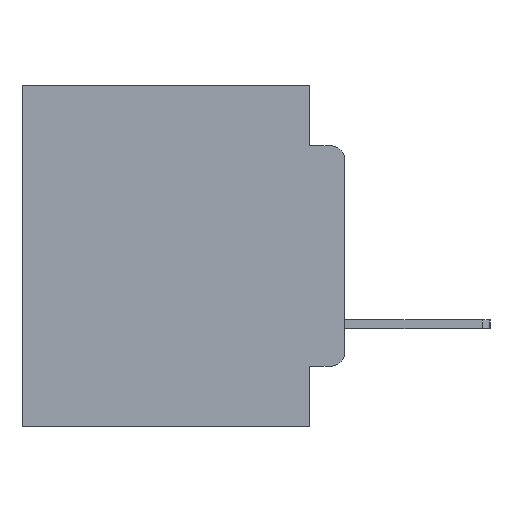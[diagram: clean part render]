
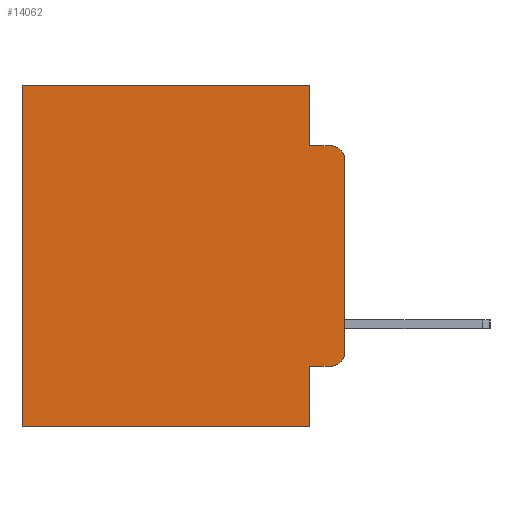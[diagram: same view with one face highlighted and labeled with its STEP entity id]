
A CAD part, left-side view. The second image highlights one B-rep face of the part: STEP entity #14062.
In plain terms, the highlighted planar face has unit normal (-1, 0, 0).
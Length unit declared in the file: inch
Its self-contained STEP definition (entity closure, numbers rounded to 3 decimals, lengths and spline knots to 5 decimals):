
#176 = VERTEX_POINT ( 'NONE', #15971 ) ;
#341 = LINE ( 'NONE', #25611, #21299 ) ;
#705 = EDGE_LOOP ( 'NONE', ( #4758, #1795, #12460, #17952, #14075, #7537, #6541, #7168, #8630, #8923 ) ) ;
#963 = CARTESIAN_POINT ( 'NONE',  ( 0.298, 0.051, -0.0885 ) ) ;
#1400 = EDGE_CURVE ( 'NONE', #21096, #8493, #10377, .T. ) ;
#1471 = CARTESIAN_POINT ( 'NONE',  ( 0.298, 0., -0.3915 ) ) ;
#1538 = DIRECTION ( 'NONE',  ( 0., 0., -1. ) ) ;
#1795 = ORIENTED_EDGE ( 'NONE', *, *, #18095, .T. ) ;
#2127 = DIRECTION ( 'NONE',  ( 0., -1., 0. ) ) ;
#2329 = VECTOR ( 'NONE', #8369, 39.37008 ) ;
#3346 = EDGE_CURVE ( 'NONE', #5875, #17686, #341, .T. ) ;
#3834 = CARTESIAN_POINT ( 'NONE',  ( 0.298, 0.473, 0. ) ) ;
#4711 = VECTOR ( 'NONE', #16511, 39.37008 ) ;
#4758 = ORIENTED_EDGE ( 'NONE', *, *, #12204, .F. ) ;
#5013 = DIRECTION ( 'NONE',  ( -1., 0., 0. ) ) ;
#5567 = LINE ( 'NONE', #6428, #20324 ) ;
#5639 = VECTOR ( 'NONE', #13535, 39.37008 ) ;
#5875 = VERTEX_POINT ( 'NONE', #3834 ) ;
#6010 = PLANE ( 'NONE',  #20145 ) ;
#6085 = CARTESIAN_POINT ( 'NONE',  ( 0.298, 0., 0. ) ) ;
#6158 = CARTESIAN_POINT ( 'NONE',  ( 0.298, 0.473, -0.5 ) ) ;
#6428 = CARTESIAN_POINT ( 'NONE',  ( 0.298, 0., -0.5 ) ) ;
#6541 = ORIENTED_EDGE ( 'NONE', *, *, #20149, .F. ) ;
#7168 = ORIENTED_EDGE ( 'NONE', *, *, #1400, .F. ) ;
#7441 = VECTOR ( 'NONE', #20025, 39.37008 ) ;
#7537 = ORIENTED_EDGE ( 'NONE', *, *, #3346, .T. ) ;
#8031 = CARTESIAN_POINT ( 'NONE',  ( 0.298, 0., -0.1085 ) ) ;
#8080 = LINE ( 'NONE', #6085, #2329 ) ;
#8151 = CARTESIAN_POINT ( 'NONE',  ( 0.298, 0., 0. ) ) ;
#8369 = DIRECTION ( 'NONE',  ( 0., 1., 0. ) ) ;
#8493 = VERTEX_POINT ( 'NONE', #16920 ) ;
#8630 = ORIENTED_EDGE ( 'NONE', *, *, #26521, .T. ) ;
#8894 = EDGE_CURVE ( 'NONE', #24601, #5875, #8080, .T. ) ;
#8923 = ORIENTED_EDGE ( 'NONE', *, *, #22632, .T. ) ;
#9739 = VECTOR ( 'NONE', #1538, 39.37008 ) ;
#10377 = LINE ( 'NONE', #15808, #9739 ) ;
#10493 = DIRECTION ( 'NONE',  ( 1., 0., 0. ) ) ;
#12106 = DIRECTION ( 'NONE',  ( -1., 0., 0. ) ) ;
#12204 = EDGE_CURVE ( 'NONE', #18691, #22281, #26534, .T. ) ;
#12460 = ORIENTED_EDGE ( 'NONE', *, *, #13393, .F. ) ;
#12464 = EDGE_CURVE ( 'NONE', #24601, #19122, #13038, .T. ) ;
#12596 = FACE_OUTER_BOUND ( 'NONE', #705, .T. ) ;
#13038 = LINE ( 'NONE', #19939, #7441 ) ;
#13225 = CARTESIAN_POINT ( 'NONE',  ( 0.298, 0.051, -0.4115 ) ) ;
#13393 = EDGE_CURVE ( 'NONE', #19122, #176, #15528, .T. ) ;
#13535 = DIRECTION ( 'NONE',  ( 0., -1., 0. ) ) ;
#14062 = ADVANCED_FACE ( 'NONE', ( #12596 ), #6010, .F. ) ;
#14075 = ORIENTED_EDGE ( 'NONE', *, *, #8894, .T. ) ;
#14567 = CARTESIAN_POINT ( 'NONE',  ( 0.298, 0.051, 0. ) ) ;
#15528 = LINE ( 'NONE', #963, #5639 ) ;
#15808 = CARTESIAN_POINT ( 'NONE',  ( 0.298, 0.051, 0. ) ) ;
#15971 = CARTESIAN_POINT ( 'NONE',  ( 0.298, 0.02, -0.0885 ) ) ;
#16511 = DIRECTION ( 'NONE',  ( 0., 0., -1. ) ) ;
#16920 = CARTESIAN_POINT ( 'NONE',  ( 0.298, 0.051, -0.5 ) ) ;
#17035 = VECTOR ( 'NONE', #2127, 39.37008 ) ;
#17651 = CARTESIAN_POINT ( 'NONE',  ( 0.298, 0.02, -0.3915 ) ) ;
#17686 = VERTEX_POINT ( 'NONE', #6158 ) ;
#17863 = AXIS2_PLACEMENT_3D ( 'NONE', #24234, #12106, #26146 ) ;
#17952 = ORIENTED_EDGE ( 'NONE', *, *, #12464, .F. ) ;
#18095 = EDGE_CURVE ( 'NONE', #18691, #176, #24251, .T. ) ;
#18298 = CARTESIAN_POINT ( 'NONE',  ( 0.298, 0.051, -0.0885 ) ) ;
#18420 = CARTESIAN_POINT ( 'NONE',  ( 0.298, 0.02, -0.4115 ) ) ;
#18691 = VERTEX_POINT ( 'NONE', #8031 ) ;
#18923 = CARTESIAN_POINT ( 'NONE',  ( 0.298, 0.051, -0.4115 ) ) ;
#19122 = VERTEX_POINT ( 'NONE', #18298 ) ;
#19738 = DIRECTION ( 'NONE',  ( 0., 0., -1. ) ) ;
#19848 = AXIS2_PLACEMENT_3D ( 'NONE', #17651, #5013, #19738 ) ;
#19939 = CARTESIAN_POINT ( 'NONE',  ( 0.298, 0.051, 0. ) ) ;
#20025 = DIRECTION ( 'NONE',  ( 0., 0., -1. ) ) ;
#20145 = AXIS2_PLACEMENT_3D ( 'NONE', #22769, #10493, #24716 ) ;
#20149 = EDGE_CURVE ( 'NONE', #8493, #17686, #5567, .T. ) ;
#20324 = VECTOR ( 'NONE', #22965, 39.37008 ) ;
#20533 = CIRCLE ( 'NONE', #19848, 0.02 ) ;
#20694 = VERTEX_POINT ( 'NONE', #18420 ) ;
#21096 = VERTEX_POINT ( 'NONE', #13225 ) ;
#21299 = VECTOR ( 'NONE', #25579, 39.37008 ) ;
#22281 = VERTEX_POINT ( 'NONE', #1471 ) ;
#22632 = EDGE_CURVE ( 'NONE', #20694, #22281, #20533, .T. ) ;
#22769 = CARTESIAN_POINT ( 'NONE',  ( 0.298, 0., 0. ) ) ;
#22965 = DIRECTION ( 'NONE',  ( 0., 1., 0. ) ) ;
#23053 = LINE ( 'NONE', #18923, #17035 ) ;
#24234 = CARTESIAN_POINT ( 'NONE',  ( 0.298, 0.02, -0.1085 ) ) ;
#24251 = CIRCLE ( 'NONE', #17863, 0.02 ) ;
#24601 = VERTEX_POINT ( 'NONE', #14567 ) ;
#24716 = DIRECTION ( 'NONE',  ( 0., 0., -1. ) ) ;
#25579 = DIRECTION ( 'NONE',  ( 0., 0., -1. ) ) ;
#25611 = CARTESIAN_POINT ( 'NONE',  ( 0.298, 0.473, 0. ) ) ;
#26146 = DIRECTION ( 'NONE',  ( 0., 0., -1. ) ) ;
#26521 = EDGE_CURVE ( 'NONE', #21096, #20694, #23053, .T. ) ;
#26534 = LINE ( 'NONE', #8151, #4711 ) ;
